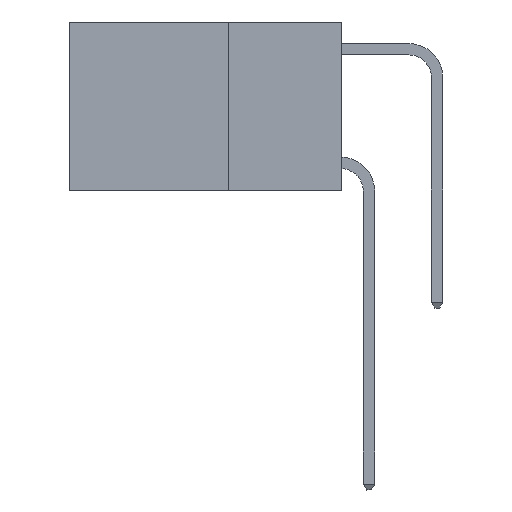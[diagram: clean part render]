
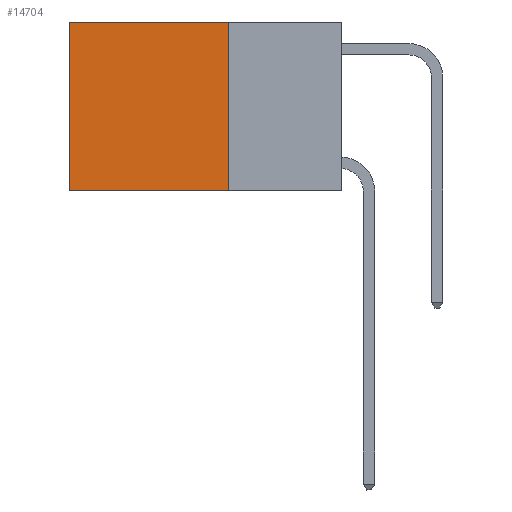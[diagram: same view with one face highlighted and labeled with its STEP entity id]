
A CAD part, left-side view. The second image highlights one B-rep face of the part: STEP entity #14704.
In plain terms, the highlighted planar face has unit normal (-1, 0, 0).
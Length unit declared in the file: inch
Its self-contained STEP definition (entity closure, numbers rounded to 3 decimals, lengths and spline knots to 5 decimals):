
#893 = VERTEX_POINT ( 'NONE', #7023 ) ;
#1913 = LINE ( 'NONE', #9000, #5942 ) ;
#2195 = CARTESIAN_POINT ( 'NONE',  ( 0.2625, 0.25, 0. ) ) ;
#2284 = CARTESIAN_POINT ( 'NONE',  ( 0.2625, 0.25, 0. ) ) ;
#2951 = DIRECTION ( 'NONE',  ( 0., 1., 0. ) ) ;
#3271 = CARTESIAN_POINT ( 'NONE',  ( 0.2625, 0.6, -0.37 ) ) ;
#3390 = CARTESIAN_POINT ( 'NONE',  ( 0.2625, 0.25, 0. ) ) ;
#3443 = ORIENTED_EDGE ( 'NONE', *, *, #11822, .T. ) ;
#3583 = FACE_OUTER_BOUND ( 'NONE', #13799, .T. ) ;
#4922 = CARTESIAN_POINT ( 'NONE',  ( 0.2625, 0.25, -0.37 ) ) ;
#5294 = EDGE_CURVE ( 'NONE', #893, #12352, #1913, .T. ) ;
#5494 = VERTEX_POINT ( 'NONE', #13997 ) ;
#5942 = VECTOR ( 'NONE', #6311, 39.37008 ) ;
#6311 = DIRECTION ( 'NONE',  ( 0., 0., -1. ) ) ;
#6911 = VECTOR ( 'NONE', #2951, 39.37008 ) ;
#7023 = CARTESIAN_POINT ( 'NONE',  ( 0.2625, 0.6, 0. ) ) ;
#7807 = DIRECTION ( 'NONE',  ( 1., 0., 0. ) ) ;
#8970 = ORIENTED_EDGE ( 'NONE', *, *, #14919, .F. ) ;
#9000 = CARTESIAN_POINT ( 'NONE',  ( 0.2625, 0.6, 0. ) ) ;
#9200 = PLANE ( 'NONE',  #11702 ) ;
#9856 = LINE ( 'NONE', #15330, #6911 ) ;
#10207 = LINE ( 'NONE', #3390, #11717 ) ;
#11140 = DIRECTION ( 'NONE',  ( 0., 0., -1. ) ) ;
#11702 = AXIS2_PLACEMENT_3D ( 'NONE', #2195, #7807, #11140 ) ;
#11717 = VECTOR ( 'NONE', #14387, 39.37008 ) ;
#11822 = EDGE_CURVE ( 'NONE', #16718, #893, #9856, .T. ) ;
#11933 = LINE ( 'NONE', #4922, #15874 ) ;
#12352 = VERTEX_POINT ( 'NONE', #3271 ) ;
#13409 = DIRECTION ( 'NONE',  ( 0., 1., 0. ) ) ;
#13799 = EDGE_LOOP ( 'NONE', ( #15926, #16742, #8970, #3443 ) ) ;
#13997 = CARTESIAN_POINT ( 'NONE',  ( 0.2625, 0.25, -0.37 ) ) ;
#14387 = DIRECTION ( 'NONE',  ( 0., 0., -1. ) ) ;
#14704 = ADVANCED_FACE ( 'NONE', ( #3583 ), #9200, .F. ) ;
#14919 = EDGE_CURVE ( 'NONE', #16718, #5494, #10207, .T. ) ;
#15157 = EDGE_CURVE ( 'NONE', #5494, #12352, #11933, .T. ) ;
#15330 = CARTESIAN_POINT ( 'NONE',  ( 0.2625, 0.25, 0. ) ) ;
#15874 = VECTOR ( 'NONE', #13409, 39.37008 ) ;
#15926 = ORIENTED_EDGE ( 'NONE', *, *, #5294, .T. ) ;
#16718 = VERTEX_POINT ( 'NONE', #2284 ) ;
#16742 = ORIENTED_EDGE ( 'NONE', *, *, #15157, .F. ) ;
